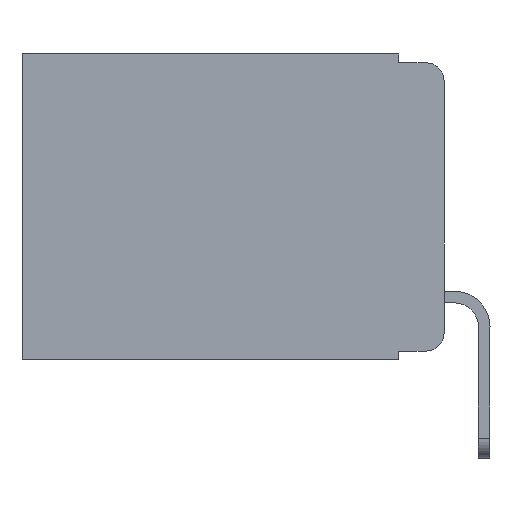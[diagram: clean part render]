
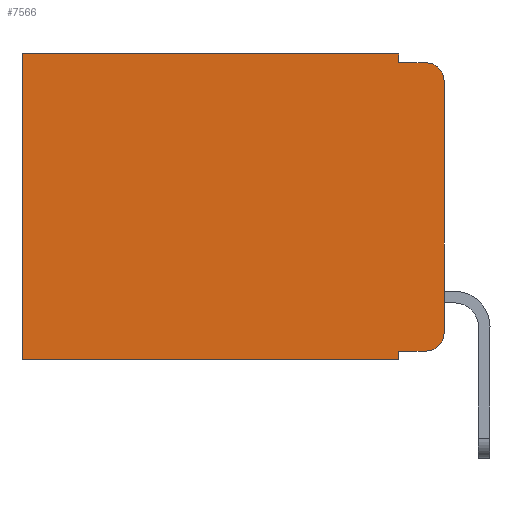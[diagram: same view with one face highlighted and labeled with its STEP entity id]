
A CAD part, left-side view. The second image highlights one B-rep face of the part: STEP entity #7566.
In plain terms, the highlighted planar face has unit normal (-1, 0, 0).
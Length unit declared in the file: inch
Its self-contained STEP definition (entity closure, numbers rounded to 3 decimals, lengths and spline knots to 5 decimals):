
#107 = LINE ( 'NONE', #10132, #17042 ) ;
#146 = EDGE_CURVE ( 'NONE', #2876, #11753, #13499, .T. ) ;
#499 = EDGE_CURVE ( 'NONE', #12985, #2876, #3356, .T. ) ;
#1067 = ORIENTED_EDGE ( 'NONE', *, *, #146, .T. ) ;
#1074 = CARTESIAN_POINT ( 'NONE',  ( 0.298, 0.051, -0.01 ) ) ;
#1919 = VECTOR ( 'NONE', #11776, 39.37008 ) ;
#2079 = VERTEX_POINT ( 'NONE', #10725 ) ;
#2144 = ORIENTED_EDGE ( 'NONE', *, *, #4359, .F. ) ;
#2213 = LINE ( 'NONE', #8146, #4860 ) ;
#2460 = VECTOR ( 'NONE', #9167, 39.37008 ) ;
#2490 = CARTESIAN_POINT ( 'NONE',  ( 0.298, 0.02, -0.333 ) ) ;
#2788 = ORIENTED_EDGE ( 'NONE', *, *, #8865, .T. ) ;
#2876 = VERTEX_POINT ( 'NONE', #2490 ) ;
#2939 = EDGE_CURVE ( 'NONE', #12711, #16346, #2213, .T. ) ;
#2950 = EDGE_CURVE ( 'NONE', #12985, #13295, #12124, .T. ) ;
#3093 = PLANE ( 'NONE',  #8522 ) ;
#3144 = VERTEX_POINT ( 'NONE', #12020 ) ;
#3155 = CARTESIAN_POINT ( 'NONE',  ( 0.298, 0., -0.03 ) ) ;
#3356 = LINE ( 'NONE', #17668, #2460 ) ;
#3386 = CARTESIAN_POINT ( 'NONE',  ( 0.298, 0.051, -0.333 ) ) ;
#3775 = CARTESIAN_POINT ( 'NONE',  ( 0.298, 0.02, -0.313 ) ) ;
#3981 = CARTESIAN_POINT ( 'NONE',  ( 0.298, 0., -0.343 ) ) ;
#4015 = CARTESIAN_POINT ( 'NONE',  ( 0.298, 0., -0.313 ) ) ;
#4357 = DIRECTION ( 'NONE',  ( 0., 0., -1. ) ) ;
#4359 = EDGE_CURVE ( 'NONE', #16346, #7363, #13365, .T. ) ;
#4418 = CARTESIAN_POINT ( 'NONE',  ( 0.298, 0.473, 0. ) ) ;
#4457 = FACE_OUTER_BOUND ( 'NONE', #17192, .T. ) ;
#4791 = VECTOR ( 'NONE', #12343, 39.37008 ) ;
#4860 = VECTOR ( 'NONE', #18090, 39.37008 ) ;
#4874 = ORIENTED_EDGE ( 'NONE', *, *, #15509, .T. ) ;
#5634 = AXIS2_PLACEMENT_3D ( 'NONE', #3775, #12393, #9383 ) ;
#5818 = CARTESIAN_POINT ( 'NONE',  ( 0.298, 0.051, -0.01 ) ) ;
#7136 = EDGE_CURVE ( 'NONE', #14881, #11753, #107, .T. ) ;
#7363 = VERTEX_POINT ( 'NONE', #11011 ) ;
#7440 = DIRECTION ( 'NONE',  ( 0., 0., -1. ) ) ;
#7482 = DIRECTION ( 'NONE',  ( -1., 0., 0. ) ) ;
#7566 = ADVANCED_FACE ( 'NONE', ( #4457 ), #3093, .F. ) ;
#8146 = CARTESIAN_POINT ( 'NONE',  ( 0.298, 0.051, 0. ) ) ;
#8522 = AXIS2_PLACEMENT_3D ( 'NONE', #11744, #10286, #7440 ) ;
#8667 = VECTOR ( 'NONE', #15166, 39.37008 ) ;
#8865 = EDGE_CURVE ( 'NONE', #2079, #3144, #16091, .T. ) ;
#8932 = DIRECTION ( 'NONE',  ( 0., 0., -1. ) ) ;
#9167 = DIRECTION ( 'NONE',  ( 0., -1., 0. ) ) ;
#9383 = DIRECTION ( 'NONE',  ( 0., 0., -1. ) ) ;
#9465 = ORIENTED_EDGE ( 'NONE', *, *, #2939, .F. ) ;
#9537 = LINE ( 'NONE', #3981, #8667 ) ;
#9640 = CIRCLE ( 'NONE', #14749, 0.02 ) ;
#10131 = ORIENTED_EDGE ( 'NONE', *, *, #7136, .F. ) ;
#10132 = CARTESIAN_POINT ( 'NONE',  ( 0.298, 0., 0. ) ) ;
#10286 = DIRECTION ( 'NONE',  ( 1., 0., 0. ) ) ;
#10725 = CARTESIAN_POINT ( 'NONE',  ( 0.298, 0.473, 0. ) ) ;
#10791 = CARTESIAN_POINT ( 'NONE',  ( 0.298, 0.051, -0.343 ) ) ;
#10911 = CARTESIAN_POINT ( 'NONE',  ( 0.298, 0.051, 0. ) ) ;
#11011 = CARTESIAN_POINT ( 'NONE',  ( 0.298, 0.02, -0.01 ) ) ;
#11156 = ORIENTED_EDGE ( 'NONE', *, *, #2950, .F. ) ;
#11228 = VECTOR ( 'NONE', #18032, 39.37008 ) ;
#11744 = CARTESIAN_POINT ( 'NONE',  ( 0.298, 0., 0. ) ) ;
#11753 = VERTEX_POINT ( 'NONE', #4015 ) ;
#11776 = DIRECTION ( 'NONE',  ( 0., 1., 0. ) ) ;
#12020 = CARTESIAN_POINT ( 'NONE',  ( 0.298, 0.473, -0.343 ) ) ;
#12058 = EDGE_CURVE ( 'NONE', #13295, #3144, #9537, .T. ) ;
#12124 = LINE ( 'NONE', #10911, #11228 ) ;
#12192 = CARTESIAN_POINT ( 'NONE',  ( 0.298, 0.051, 0. ) ) ;
#12343 = DIRECTION ( 'NONE',  ( 0., -1., 0. ) ) ;
#12393 = DIRECTION ( 'NONE',  ( -1., 0., 0. ) ) ;
#12711 = VERTEX_POINT ( 'NONE', #12192 ) ;
#12723 = LINE ( 'NONE', #17520, #1919 ) ;
#12954 = DIRECTION ( 'NONE',  ( 0., 0., -1. ) ) ;
#12985 = VERTEX_POINT ( 'NONE', #3386 ) ;
#13295 = VERTEX_POINT ( 'NONE', #10791 ) ;
#13365 = LINE ( 'NONE', #1074, #4791 ) ;
#13499 = CIRCLE ( 'NONE', #5634, 0.02 ) ;
#13611 = ORIENTED_EDGE ( 'NONE', *, *, #499, .T. ) ;
#14386 = CARTESIAN_POINT ( 'NONE',  ( 0.298, 0.02, -0.03 ) ) ;
#14749 = AXIS2_PLACEMENT_3D ( 'NONE', #14386, #7482, #8932 ) ;
#14881 = VERTEX_POINT ( 'NONE', #3155 ) ;
#15075 = ORIENTED_EDGE ( 'NONE', *, *, #16424, .T. ) ;
#15166 = DIRECTION ( 'NONE',  ( 0., 1., 0. ) ) ;
#15509 = EDGE_CURVE ( 'NONE', #14881, #7363, #9640, .T. ) ;
#16091 = LINE ( 'NONE', #4418, #17425 ) ;
#16346 = VERTEX_POINT ( 'NONE', #5818 ) ;
#16424 = EDGE_CURVE ( 'NONE', #12711, #2079, #12723, .T. ) ;
#17042 = VECTOR ( 'NONE', #12954, 39.37008 ) ;
#17192 = EDGE_LOOP ( 'NONE', ( #10131, #4874, #2144, #9465, #15075, #2788, #17328, #11156, #13611, #1067 ) ) ;
#17328 = ORIENTED_EDGE ( 'NONE', *, *, #12058, .F. ) ;
#17425 = VECTOR ( 'NONE', #4357, 39.37008 ) ;
#17520 = CARTESIAN_POINT ( 'NONE',  ( 0.298, 0., 0. ) ) ;
#17668 = CARTESIAN_POINT ( 'NONE',  ( 0.298, 0.051, -0.333 ) ) ;
#18032 = DIRECTION ( 'NONE',  ( 0., 0., -1. ) ) ;
#18090 = DIRECTION ( 'NONE',  ( 0., 0., -1. ) ) ;
